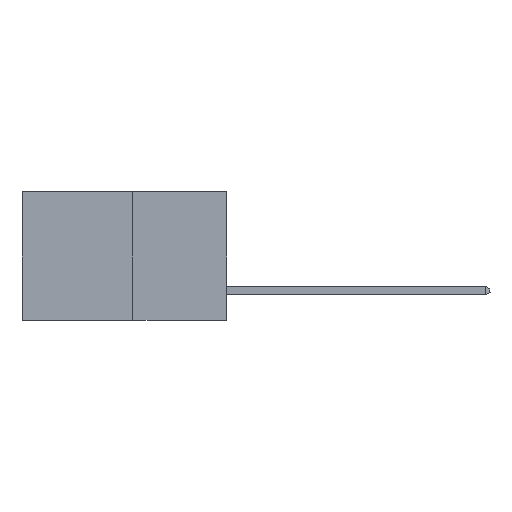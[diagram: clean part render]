
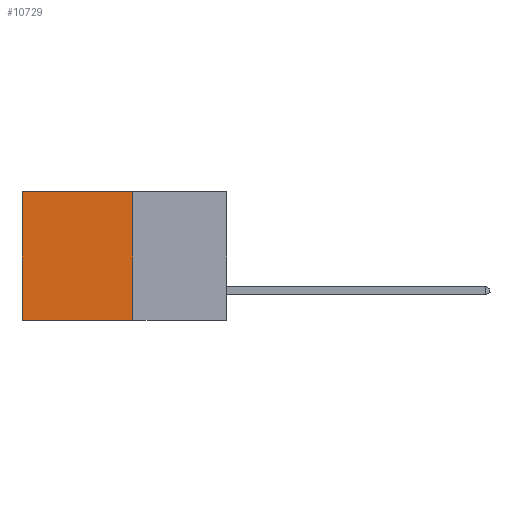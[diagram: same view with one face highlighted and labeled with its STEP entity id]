
A CAD part, left-side view. The second image highlights one B-rep face of the part: STEP entity #10729.
In plain terms, the highlighted planar face has unit normal (-1, 0, 0).
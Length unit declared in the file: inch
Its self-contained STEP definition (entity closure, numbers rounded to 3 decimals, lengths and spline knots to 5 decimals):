
#640 = DIRECTION ( 'NONE',  ( 0., 0., -1. ) ) ;
#3313 = EDGE_LOOP ( 'NONE', ( #17524, #5596, #3968, #4299 ) ) ;
#3968 = ORIENTED_EDGE ( 'NONE', *, *, #10081, .F. ) ;
#4299 = ORIENTED_EDGE ( 'NONE', *, *, #28167, .T. ) ;
#4786 = VECTOR ( 'NONE', #10305, 39.37008 ) ;
#4904 = LINE ( 'NONE', #12668, #22370 ) ;
#5495 = LINE ( 'NONE', #21671, #4786 ) ;
#5596 = ORIENTED_EDGE ( 'NONE', *, *, #16376, .F. ) ;
#6817 = CARTESIAN_POINT ( 'NONE',  ( 0.277, 0.27, 0. ) ) ;
#7364 = CARTESIAN_POINT ( 'NONE',  ( 0.277, 0.59, -0.37 ) ) ;
#8133 = EDGE_CURVE ( 'NONE', #18231, #28227, #23716, .T. ) ;
#8993 = LINE ( 'NONE', #27792, #21813 ) ;
#10081 = EDGE_CURVE ( 'NONE', #23807, #16604, #5495, .T. ) ;
#10305 = DIRECTION ( 'NONE',  ( 0., 0., -1. ) ) ;
#10729 = ADVANCED_FACE ( 'NONE', ( #19122 ), #25976, .F. ) ;
#11187 = CARTESIAN_POINT ( 'NONE',  ( 0.277, 0.27, -0.37 ) ) ;
#11613 = VECTOR ( 'NONE', #640, 39.37008 ) ;
#12668 = CARTESIAN_POINT ( 'NONE',  ( 0.277, 0.27, -0.37 ) ) ;
#14119 = DIRECTION ( 'NONE',  ( 0., 1., 0. ) ) ;
#14723 = DIRECTION ( 'NONE',  ( 0., 0., -1. ) ) ;
#14960 = DIRECTION ( 'NONE',  ( 0., 1., 0. ) ) ;
#16376 = EDGE_CURVE ( 'NONE', #16604, #28227, #4904, .T. ) ;
#16604 = VERTEX_POINT ( 'NONE', #11187 ) ;
#16625 = CARTESIAN_POINT ( 'NONE',  ( 0.277, 0.59, -0.37 ) ) ;
#17524 = ORIENTED_EDGE ( 'NONE', *, *, #8133, .T. ) ;
#18231 = VERTEX_POINT ( 'NONE', #18654 ) ;
#18654 = CARTESIAN_POINT ( 'NONE',  ( 0.277, 0.59, 0. ) ) ;
#19122 = FACE_OUTER_BOUND ( 'NONE', #3313, .T. ) ;
#21671 = CARTESIAN_POINT ( 'NONE',  ( 0.277, 0.27, -0.37 ) ) ;
#21813 = VECTOR ( 'NONE', #14119, 39.37008 ) ;
#22370 = VECTOR ( 'NONE', #14960, 39.37008 ) ;
#22723 = AXIS2_PLACEMENT_3D ( 'NONE', #26077, #28398, #14723 ) ;
#23716 = LINE ( 'NONE', #7364, #11613 ) ;
#23807 = VERTEX_POINT ( 'NONE', #6817 ) ;
#25976 = PLANE ( 'NONE',  #22723 ) ;
#26077 = CARTESIAN_POINT ( 'NONE',  ( 0.277, 0.27, -0.37 ) ) ;
#27792 = CARTESIAN_POINT ( 'NONE',  ( 0.277, 0.27, 0. ) ) ;
#28167 = EDGE_CURVE ( 'NONE', #23807, #18231, #8993, .T. ) ;
#28227 = VERTEX_POINT ( 'NONE', #16625 ) ;
#28398 = DIRECTION ( 'NONE',  ( 1., 0., 0. ) ) ;
